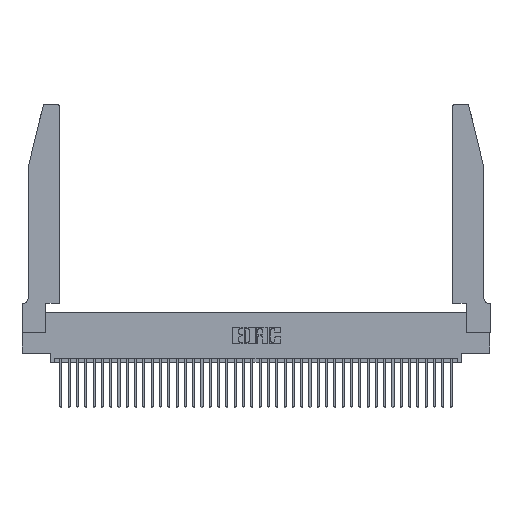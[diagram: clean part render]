
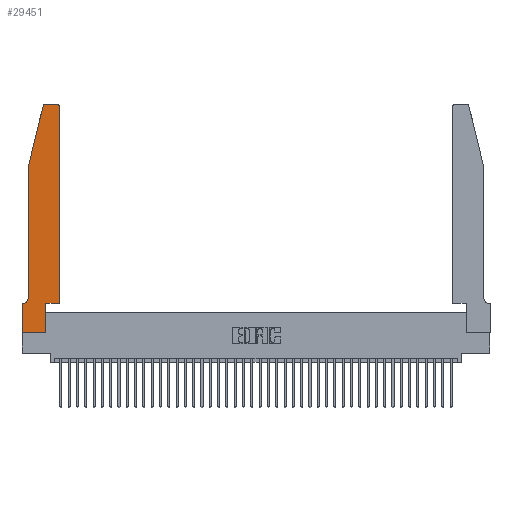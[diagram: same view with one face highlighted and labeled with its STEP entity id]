
A CAD part, top view. The second image highlights one B-rep face of the part: STEP entity #29451.
In plain terms, the highlighted planar face has unit normal (0, 0, 1).
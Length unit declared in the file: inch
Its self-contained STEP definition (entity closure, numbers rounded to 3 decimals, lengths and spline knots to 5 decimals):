
#993 = EDGE_CURVE ( 'NONE', #16160, #11252, #7596, .T. ) ;
#1925 = DIRECTION ( 'NONE',  ( 0., -1., 0. ) ) ;
#2017 = CARTESIAN_POINT ( 'NONE',  ( 0.0755, 0.42, 0.37 ) ) ;
#2129 = ORIENTED_EDGE ( 'NONE', *, *, #37326, .T. ) ;
#2156 = EDGE_CURVE ( 'NONE', #12215, #34087, #34894, .T. ) ;
#2396 = VECTOR ( 'NONE', #8709, 39.37008 ) ;
#3328 = CARTESIAN_POINT ( 'NONE',  ( 0.0755, 0.35, 0.37 ) ) ;
#3761 = AXIS2_PLACEMENT_3D ( 'NONE', #19169, #41428, #22444 ) ;
#4479 = PLANE ( 'NONE',  #26518 ) ;
#5884 = ORIENTED_EDGE ( 'NONE', *, *, #22055, .T. ) ;
#6060 = VECTOR ( 'NONE', #8048, 39.37008 ) ;
#6621 = DIRECTION ( 'NONE',  ( -1., 0., 0. ) ) ;
#7123 = CIRCLE ( 'NONE', #16373, 0.03 ) ;
#7596 = CIRCLE ( 'NONE', #27495, 0.03 ) ;
#7751 = DIRECTION ( 'NONE',  ( 1., 0., 0. ) ) ;
#7855 = VECTOR ( 'NONE', #6621, 39.37008 ) ;
#8048 = DIRECTION ( 'NONE',  ( 0., -1., 0. ) ) ;
#8252 = CARTESIAN_POINT ( 'NONE',  ( 0.4205, 2.75, 0.37 ) ) ;
#8709 = DIRECTION ( 'NONE',  ( 1., 0., 0. ) ) ;
#8749 = CARTESIAN_POINT ( 'NONE',  ( 0., 0., 0.37 ) ) ;
#8975 = LINE ( 'NONE', #31839, #25266 ) ;
#9061 = CARTESIAN_POINT ( 'NONE',  ( 0.4205, 2.72, 0.37 ) ) ;
#9292 = VERTEX_POINT ( 'NONE', #32155 ) ;
#9485 = CARTESIAN_POINT ( 'NONE',  ( 0., 0.35, 0.37 ) ) ;
#11129 = LINE ( 'NONE', #40749, #2396 ) ;
#11252 = VERTEX_POINT ( 'NONE', #8252 ) ;
#11844 = EDGE_CURVE ( 'NONE', #15678, #14345, #35533, .T. ) ;
#12215 = VERTEX_POINT ( 'NONE', #9485 ) ;
#12227 = EDGE_LOOP ( 'NONE', ( #36675, #29685, #20215, #32781, #30580, #5884, #14097, #35669, #2129, #41405, #20567, #16729 ) ) ;
#12351 = DIRECTION ( 'NONE',  ( 1., 0., 0. ) ) ;
#12545 = VERTEX_POINT ( 'NONE', #14761 ) ;
#13967 = LINE ( 'NONE', #21723, #30111 ) ;
#14097 = ORIENTED_EDGE ( 'NONE', *, *, #2156, .T. ) ;
#14345 = VERTEX_POINT ( 'NONE', #37909 ) ;
#14387 = CARTESIAN_POINT ( 'NONE',  ( 0.0755, 2., 0.37 ) ) ;
#14761 = CARTESIAN_POINT ( 'NONE',  ( 0.4505, 0.35, 0.37 ) ) ;
#14774 = LINE ( 'NONE', #30694, #6060 ) ;
#14980 = EDGE_CURVE ( 'NONE', #31438, #12545, #11129, .T. ) ;
#15656 = VECTOR ( 'NONE', #32245, 39.37008 ) ;
#15678 = VERTEX_POINT ( 'NONE', #40556 ) ;
#16160 = VERTEX_POINT ( 'NONE', #41506 ) ;
#16373 = AXIS2_PLACEMENT_3D ( 'NONE', #19089, #41353, #22369 ) ;
#16729 = ORIENTED_EDGE ( 'NONE', *, *, #993, .T. ) ;
#18515 = VECTOR ( 'NONE', #24192, 39.37008 ) ;
#19034 = CARTESIAN_POINT ( 'NONE',  ( 0.284, 2.75, 0.37 ) ) ;
#19089 = CARTESIAN_POINT ( 'NONE',  ( 0.284, 2.72, 0.37 ) ) ;
#19169 = CARTESIAN_POINT ( 'NONE',  ( 0.0055, 0.42, 0.37 ) ) ;
#20215 = ORIENTED_EDGE ( 'NONE', *, *, #11844, .T. ) ;
#20567 = ORIENTED_EDGE ( 'NONE', *, *, #32753, .T. ) ;
#20752 = EDGE_CURVE ( 'NONE', #40975, #15678, #7123, .T. ) ;
#20779 = CARTESIAN_POINT ( 'NONE',  ( 0., 0.35, 0.37 ) ) ;
#21723 = CARTESIAN_POINT ( 'NONE',  ( 0.2605, 2.75, 0.37 ) ) ;
#22055 = EDGE_CURVE ( 'NONE', #9292, #12215, #25171, .T. ) ;
#22369 = DIRECTION ( 'NONE',  ( 1., 0., 0. ) ) ;
#22444 = DIRECTION ( 'NONE',  ( -1., 0., 0. ) ) ;
#23293 = LINE ( 'NONE', #38585, #15656 ) ;
#23790 = VERTEX_POINT ( 'NONE', #28592 ) ;
#24192 = DIRECTION ( 'NONE',  ( -0.239, -0.971, 0. ) ) ;
#24932 = DIRECTION ( 'NONE',  ( -1., 0., 0. ) ) ;
#24974 = EDGE_CURVE ( 'NONE', #14345, #30840, #14774, .T. ) ;
#25171 = LINE ( 'NONE', #3328, #7855 ) ;
#25266 = VECTOR ( 'NONE', #35020, 39.37008 ) ;
#25284 = LINE ( 'NONE', #35190, #32775 ) ;
#25411 = VECTOR ( 'NONE', #1925, 39.37008 ) ;
#26518 = AXIS2_PLACEMENT_3D ( 'NONE', #20779, #27159, #7751 ) ;
#27159 = DIRECTION ( 'NONE',  ( 0., 0., 1. ) ) ;
#27495 = AXIS2_PLACEMENT_3D ( 'NONE', #9061, #31691, #12351 ) ;
#27549 = EDGE_CURVE ( 'NONE', #11252, #40975, #13967, .T. ) ;
#28592 = CARTESIAN_POINT ( 'NONE',  ( 0.2865, 0., 0.37 ) ) ;
#28942 = FACE_OUTER_BOUND ( 'NONE', #12227, .T. ) ;
#29451 = ADVANCED_FACE ( 'NONE', ( #28942 ), #4479, .T. ) ;
#29685 = ORIENTED_EDGE ( 'NONE', *, *, #20752, .T. ) ;
#30111 = VECTOR ( 'NONE', #24932, 39.37008 ) ;
#30580 = ORIENTED_EDGE ( 'NONE', *, *, #33464, .T. ) ;
#30694 = CARTESIAN_POINT ( 'NONE',  ( 0.0755, 2., 0.37 ) ) ;
#30840 = VERTEX_POINT ( 'NONE', #2017 ) ;
#31438 = VERTEX_POINT ( 'NONE', #34423 ) ;
#31691 = DIRECTION ( 'NONE',  ( 0., 0., 1. ) ) ;
#31839 = CARTESIAN_POINT ( 'NONE',  ( 0.4505, 0.35, 0.37 ) ) ;
#32155 = CARTESIAN_POINT ( 'NONE',  ( 0.0055, 0.35, 0.37 ) ) ;
#32245 = DIRECTION ( 'NONE',  ( 1., 0., 0. ) ) ;
#32753 = EDGE_CURVE ( 'NONE', #12545, #16160, #8975, .T. ) ;
#32775 = VECTOR ( 'NONE', #38370, 39.37008 ) ;
#32781 = ORIENTED_EDGE ( 'NONE', *, *, #24974, .T. ) ;
#33464 = EDGE_CURVE ( 'NONE', #30840, #9292, #40573, .T. ) ;
#34087 = VERTEX_POINT ( 'NONE', #8749 ) ;
#34423 = CARTESIAN_POINT ( 'NONE',  ( 0.2865, 0.35, 0.37 ) ) ;
#34894 = LINE ( 'NONE', #37393, #25411 ) ;
#35020 = DIRECTION ( 'NONE',  ( 0., 1., 0. ) ) ;
#35190 = CARTESIAN_POINT ( 'NONE',  ( 0.2865, 0.35, 0.37 ) ) ;
#35533 = LINE ( 'NONE', #14387, #18515 ) ;
#35669 = ORIENTED_EDGE ( 'NONE', *, *, #38053, .T. ) ;
#36675 = ORIENTED_EDGE ( 'NONE', *, *, #27549, .T. ) ;
#37326 = EDGE_CURVE ( 'NONE', #23790, #31438, #25284, .T. ) ;
#37393 = CARTESIAN_POINT ( 'NONE',  ( 0., 0., 0.37 ) ) ;
#37909 = CARTESIAN_POINT ( 'NONE',  ( 0.0755, 2., 0.37 ) ) ;
#38053 = EDGE_CURVE ( 'NONE', #34087, #23790, #23293, .T. ) ;
#38370 = DIRECTION ( 'NONE',  ( 0., 1., 0. ) ) ;
#38585 = CARTESIAN_POINT ( 'NONE',  ( 0., 0., 0.37 ) ) ;
#40556 = CARTESIAN_POINT ( 'NONE',  ( 0.25487, 2.72718, 0.37 ) ) ;
#40573 = CIRCLE ( 'NONE', #3761, 0.07 ) ;
#40749 = CARTESIAN_POINT ( 'NONE',  ( 0.4505, 0.35, 0.37 ) ) ;
#40975 = VERTEX_POINT ( 'NONE', #19034 ) ;
#41353 = DIRECTION ( 'NONE',  ( 0., 0., 1. ) ) ;
#41405 = ORIENTED_EDGE ( 'NONE', *, *, #14980, .T. ) ;
#41428 = DIRECTION ( 'NONE',  ( 0., 0., -1. ) ) ;
#41506 = CARTESIAN_POINT ( 'NONE',  ( 0.4505, 2.72, 0.37 ) ) ;
